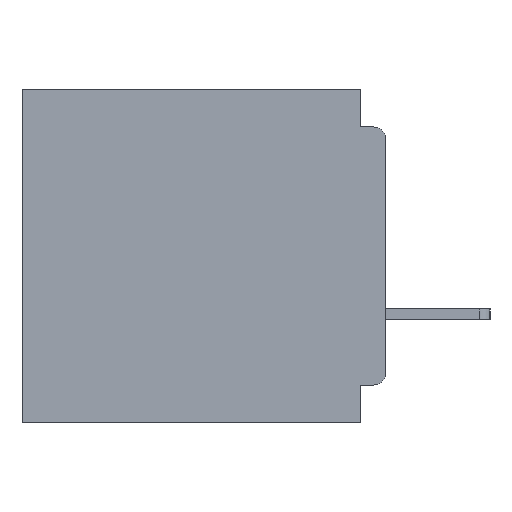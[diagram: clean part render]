
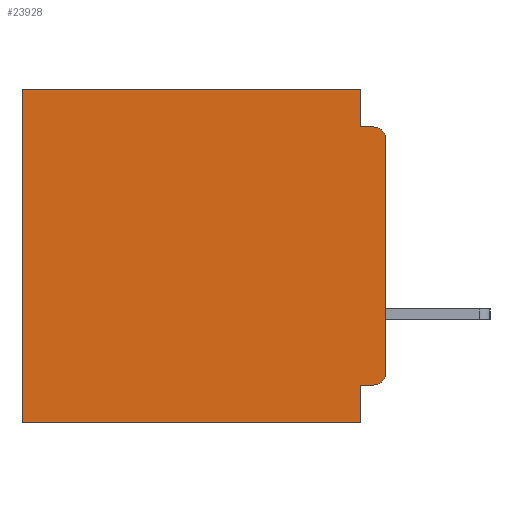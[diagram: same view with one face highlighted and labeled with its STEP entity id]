
A CAD part, left-side view. The second image highlights one B-rep face of the part: STEP entity #23928.
In plain terms, the highlighted planar face has unit normal (-1, 0, 0).
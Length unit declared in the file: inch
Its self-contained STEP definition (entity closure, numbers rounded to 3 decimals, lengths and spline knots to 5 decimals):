
#146 = CARTESIAN_POINT ( 'NONE',  ( 0.3, 0., 0. ) ) ;
#892 = CARTESIAN_POINT ( 'NONE',  ( 0.3, 0.031, -0.4 ) ) ;
#1314 = EDGE_CURVE ( 'NONE', #37328, #2700, #4610, .T. ) ;
#2426 = CARTESIAN_POINT ( 'NONE',  ( 0.3, 0.031, -0.4 ) ) ;
#2700 = VERTEX_POINT ( 'NONE', #46247 ) ;
#2720 = CARTESIAN_POINT ( 'NONE',  ( 0.3, 0.031, 0. ) ) ;
#3088 = DIRECTION ( 'NONE',  ( 0., 0., -1. ) ) ;
#3992 = EDGE_LOOP ( 'NONE', ( #17934, #31254, #10602, #39736, #45210, #42145, #48827, #32427, #41519, #20925 ) ) ;
#4001 = DIRECTION ( 'NONE',  ( 0., 1., 0. ) ) ;
#4258 = EDGE_CURVE ( 'NONE', #22084, #2700, #42682, .T. ) ;
#4576 = DIRECTION ( 'NONE',  ( 0., 0., -1. ) ) ;
#4610 = LINE ( 'NONE', #6773, #43420 ) ;
#5316 = VERTEX_POINT ( 'NONE', #46921 ) ;
#6555 = DIRECTION ( 'NONE',  ( 0., 0., -1. ) ) ;
#6773 = CARTESIAN_POINT ( 'NONE',  ( 0.3, 0.437, -0.4 ) ) ;
#8871 = DIRECTION ( 'NONE',  ( 1., 0., 0. ) ) ;
#9056 = AXIS2_PLACEMENT_3D ( 'NONE', #20481, #8871, #36035 ) ;
#10193 = LINE ( 'NONE', #22534, #28444 ) ;
#10483 = AXIS2_PLACEMENT_3D ( 'NONE', #43201, #20029, #47124 ) ;
#10602 = ORIENTED_EDGE ( 'NONE', *, *, #18642, .F. ) ;
#13193 = AXIS2_PLACEMENT_3D ( 'NONE', #13962, #41080, #17882 ) ;
#13962 = CARTESIAN_POINT ( 'NONE',  ( 0.3, 0.015, -0.34 ) ) ;
#15641 = CARTESIAN_POINT ( 'NONE',  ( 0.3, 0., -0.4 ) ) ;
#15717 = VECTOR ( 'NONE', #4576, 39.37008 ) ;
#16856 = CARTESIAN_POINT ( 'NONE',  ( 0.3, 0.015, -0.045 ) ) ;
#17226 = DIRECTION ( 'NONE',  ( 0., 0., -1. ) ) ;
#17367 = DIRECTION ( 'NONE',  ( 0., 1., 0. ) ) ;
#17882 = DIRECTION ( 'NONE',  ( 0., 0., -1. ) ) ;
#17934 = ORIENTED_EDGE ( 'NONE', *, *, #36825, .F. ) ;
#17999 = VECTOR ( 'NONE', #4001, 39.37008 ) ;
#18264 = EDGE_CURVE ( 'NONE', #21712, #22084, #28485, .T. ) ;
#18642 = EDGE_CURVE ( 'NONE', #47926, #26360, #10193, .T. ) ;
#18816 = DIRECTION ( 'NONE',  ( 0., -1., 0. ) ) ;
#19607 = EDGE_CURVE ( 'NONE', #36477, #47896, #45303, .T. ) ;
#20029 = DIRECTION ( 'NONE',  ( -1., 0., 0. ) ) ;
#20481 = CARTESIAN_POINT ( 'NONE',  ( 0.3, 0., -0.4 ) ) ;
#20887 = EDGE_CURVE ( 'NONE', #5316, #47926, #47899, .T. ) ;
#20925 = ORIENTED_EDGE ( 'NONE', *, *, #19607, .T. ) ;
#21536 = CARTESIAN_POINT ( 'NONE',  ( 0.3, 0.437, 0. ) ) ;
#21712 = VERTEX_POINT ( 'NONE', #42610 ) ;
#22084 = VERTEX_POINT ( 'NONE', #2426 ) ;
#22513 = CARTESIAN_POINT ( 'NONE',  ( 0.3, 0., -0.355 ) ) ;
#22534 = CARTESIAN_POINT ( 'NONE',  ( 0.3, 0., -0.045 ) ) ;
#23928 = ADVANCED_FACE ( 'NONE', ( #43873 ), #47584, .F. ) ;
#26318 = CARTESIAN_POINT ( 'NONE',  ( 0.3, 0., -0.4 ) ) ;
#26360 = VERTEX_POINT ( 'NONE', #16856 ) ;
#26564 = CARTESIAN_POINT ( 'NONE',  ( 0.3, 0., -0.06 ) ) ;
#27956 = CARTESIAN_POINT ( 'NONE',  ( 0.3, 0., -0.34 ) ) ;
#28444 = VECTOR ( 'NONE', #18816, 39.37008 ) ;
#28485 = LINE ( 'NONE', #892, #15717 ) ;
#28500 = VECTOR ( 'NONE', #6555, 39.37008 ) ;
#31254 = ORIENTED_EDGE ( 'NONE', *, *, #35160, .T. ) ;
#31747 = VECTOR ( 'NONE', #49659, 39.37008 ) ;
#32427 = ORIENTED_EDGE ( 'NONE', *, *, #18264, .F. ) ;
#32971 = CIRCLE ( 'NONE', #10483, 0.015 ) ;
#33516 = VERTEX_POINT ( 'NONE', #26564 ) ;
#34815 = VECTOR ( 'NONE', #17367, 39.37008 ) ;
#35160 = EDGE_CURVE ( 'NONE', #33516, #26360, #32971, .T. ) ;
#35880 = LINE ( 'NONE', #26318, #46201 ) ;
#36035 = DIRECTION ( 'NONE',  ( 0., 0., -1. ) ) ;
#36477 = VERTEX_POINT ( 'NONE', #39521 ) ;
#36825 = EDGE_CURVE ( 'NONE', #33516, #47896, #35880, .T. ) ;
#37328 = VERTEX_POINT ( 'NONE', #21536 ) ;
#38739 = EDGE_CURVE ( 'NONE', #5316, #37328, #48928, .T. ) ;
#39521 = CARTESIAN_POINT ( 'NONE',  ( 0.3, 0.015, -0.355 ) ) ;
#39736 = ORIENTED_EDGE ( 'NONE', *, *, #20887, .F. ) ;
#40352 = EDGE_CURVE ( 'NONE', #36477, #21712, #42049, .T. ) ;
#41080 = DIRECTION ( 'NONE',  ( -1., 0., 0. ) ) ;
#41519 = ORIENTED_EDGE ( 'NONE', *, *, #40352, .F. ) ;
#42049 = LINE ( 'NONE', #22513, #31747 ) ;
#42145 = ORIENTED_EDGE ( 'NONE', *, *, #1314, .T. ) ;
#42610 = CARTESIAN_POINT ( 'NONE',  ( 0.3, 0.031, -0.355 ) ) ;
#42682 = LINE ( 'NONE', #15641, #34815 ) ;
#43201 = CARTESIAN_POINT ( 'NONE',  ( 0.3, 0.015, -0.06 ) ) ;
#43420 = VECTOR ( 'NONE', #17226, 39.37008 ) ;
#43497 = CARTESIAN_POINT ( 'NONE',  ( 0.3, 0.031, -0.045 ) ) ;
#43873 = FACE_OUTER_BOUND ( 'NONE', #3992, .T. ) ;
#45210 = ORIENTED_EDGE ( 'NONE', *, *, #38739, .T. ) ;
#45303 = CIRCLE ( 'NONE', #13193, 0.015 ) ;
#46201 = VECTOR ( 'NONE', #3088, 39.37008 ) ;
#46247 = CARTESIAN_POINT ( 'NONE',  ( 0.3, 0.437, -0.4 ) ) ;
#46921 = CARTESIAN_POINT ( 'NONE',  ( 0.3, 0.031, 0. ) ) ;
#47124 = DIRECTION ( 'NONE',  ( 0., 0., -1. ) ) ;
#47584 = PLANE ( 'NONE',  #9056 ) ;
#47896 = VERTEX_POINT ( 'NONE', #27956 ) ;
#47899 = LINE ( 'NONE', #2720, #28500 ) ;
#47926 = VERTEX_POINT ( 'NONE', #43497 ) ;
#48827 = ORIENTED_EDGE ( 'NONE', *, *, #4258, .F. ) ;
#48928 = LINE ( 'NONE', #146, #17999 ) ;
#49659 = DIRECTION ( 'NONE',  ( 0., 1., 0. ) ) ;
